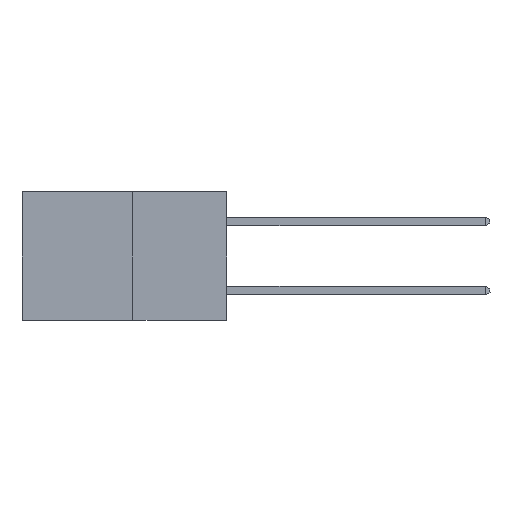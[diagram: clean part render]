
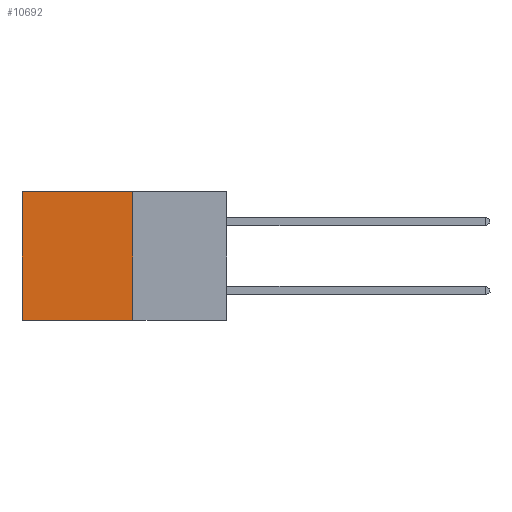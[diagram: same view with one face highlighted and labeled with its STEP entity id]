
A CAD part, left-side view. The second image highlights one B-rep face of the part: STEP entity #10692.
In plain terms, the highlighted planar face has unit normal (-1, 0, 0).
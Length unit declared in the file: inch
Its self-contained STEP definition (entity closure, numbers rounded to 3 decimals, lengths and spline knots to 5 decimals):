
#1657 = EDGE_LOOP ( 'NONE', ( #16493, #16860, #25586, #24567 ) ) ;
#1907 = DIRECTION ( 'NONE',  ( 1., 0., 0. ) ) ;
#2321 = VECTOR ( 'NONE', #31862, 39.37008 ) ;
#2784 = VECTOR ( 'NONE', #14584, 39.37008 ) ;
#3924 = EDGE_CURVE ( 'NONE', #28422, #22141, #30430, .T. ) ;
#7058 = EDGE_CURVE ( 'NONE', #7285, #22141, #22413, .T. ) ;
#7285 = VERTEX_POINT ( 'NONE', #28794 ) ;
#7298 = CARTESIAN_POINT ( 'NONE',  ( 0.277, 0.27, 0. ) ) ;
#8391 = CARTESIAN_POINT ( 'NONE',  ( 0.277, 0.27, 0. ) ) ;
#9848 = CARTESIAN_POINT ( 'NONE',  ( 0.277, 0.27, -0.37 ) ) ;
#10027 = DIRECTION ( 'NONE',  ( 0., 1., 0. ) ) ;
#10692 = ADVANCED_FACE ( 'NONE', ( #20475 ), #14448, .F. ) ;
#12076 = CARTESIAN_POINT ( 'NONE',  ( 0.277, 0.27, -0.37 ) ) ;
#13715 = LINE ( 'NONE', #8391, #14474 ) ;
#14448 = PLANE ( 'NONE',  #22659 ) ;
#14474 = VECTOR ( 'NONE', #26109, 39.37008 ) ;
#14584 = DIRECTION ( 'NONE',  ( 0., 0., -1. ) ) ;
#15221 = EDGE_CURVE ( 'NONE', #21905, #28422, #22906, .T. ) ;
#16493 = ORIENTED_EDGE ( 'NONE', *, *, #7058, .T. ) ;
#16854 = EDGE_CURVE ( 'NONE', #21905, #7285, #13715, .T. ) ;
#16860 = ORIENTED_EDGE ( 'NONE', *, *, #3924, .F. ) ;
#18158 = CARTESIAN_POINT ( 'NONE',  ( 0.277, 0.59, -0.37 ) ) ;
#19437 = CARTESIAN_POINT ( 'NONE',  ( 0.277, 0.59, -0.37 ) ) ;
#19540 = DIRECTION ( 'NONE',  ( 0., 0., -1. ) ) ;
#20475 = FACE_OUTER_BOUND ( 'NONE', #1657, .T. ) ;
#21905 = VERTEX_POINT ( 'NONE', #7298 ) ;
#22141 = VERTEX_POINT ( 'NONE', #18158 ) ;
#22413 = LINE ( 'NONE', #19437, #2321 ) ;
#22659 = AXIS2_PLACEMENT_3D ( 'NONE', #32438, #1907, #19540 ) ;
#22906 = LINE ( 'NONE', #12076, #2784 ) ;
#23455 = VECTOR ( 'NONE', #10027, 39.37008 ) ;
#24567 = ORIENTED_EDGE ( 'NONE', *, *, #16854, .T. ) ;
#25586 = ORIENTED_EDGE ( 'NONE', *, *, #15221, .F. ) ;
#26109 = DIRECTION ( 'NONE',  ( 0., 1., 0. ) ) ;
#28422 = VERTEX_POINT ( 'NONE', #31113 ) ;
#28794 = CARTESIAN_POINT ( 'NONE',  ( 0.277, 0.59, 0. ) ) ;
#30430 = LINE ( 'NONE', #9848, #23455 ) ;
#31113 = CARTESIAN_POINT ( 'NONE',  ( 0.277, 0.27, -0.37 ) ) ;
#31862 = DIRECTION ( 'NONE',  ( 0., 0., -1. ) ) ;
#32438 = CARTESIAN_POINT ( 'NONE',  ( 0.277, 0.27, -0.37 ) ) ;
